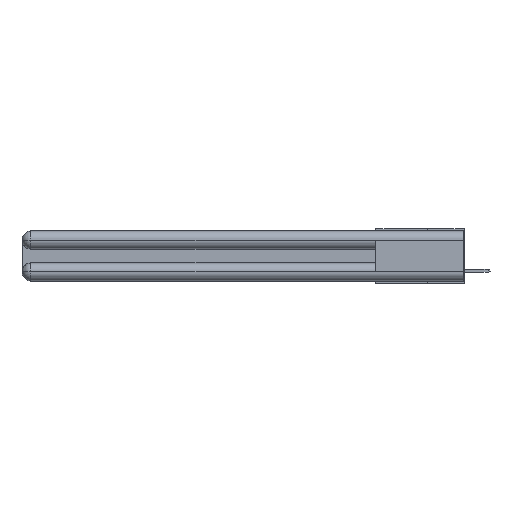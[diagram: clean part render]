
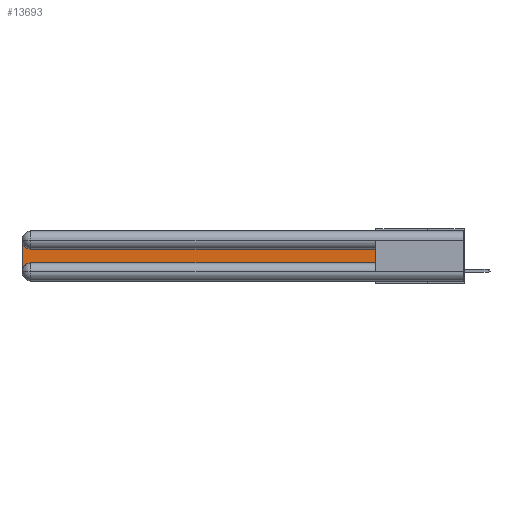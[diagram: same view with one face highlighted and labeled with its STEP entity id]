
A CAD part, left-side view. The second image highlights one B-rep face of the part: STEP entity #13693.
In plain terms, the highlighted planar face has unit normal (-1, 0, 0).
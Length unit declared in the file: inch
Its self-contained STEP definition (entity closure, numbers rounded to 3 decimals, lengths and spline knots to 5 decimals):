
#101 = CARTESIAN_POINT ( 'NONE',  ( 0.075, 2.94, -0.2175 ) ) ;
#465 = VECTOR ( 'NONE', #5358, 39.37008 ) ;
#733 = DIRECTION ( 'NONE',  ( 0., 0., -1. ) ) ;
#2989 = CARTESIAN_POINT ( 'NONE',  ( 0.075, 2.94, -0.1225 ) ) ;
#3214 = EDGE_CURVE ( 'NONE', #12078, #3903, #7138, .T. ) ;
#3518 = DIRECTION ( 'NONE',  ( 0., 0., -1. ) ) ;
#3673 = EDGE_LOOP ( 'NONE', ( #28659, #23181, #9239, #20537, #23320, #14906 ) ) ;
#3903 = VERTEX_POINT ( 'NONE', #20853 ) ;
#4995 = LINE ( 'NONE', #23506, #28482 ) ;
#5081 = DIRECTION ( 'NONE',  ( 0., 1., 0. ) ) ;
#5358 = DIRECTION ( 'NONE',  ( 0., -1., 0. ) ) ;
#6648 = EDGE_CURVE ( 'NONE', #18941, #13173, #21908, .T. ) ;
#7138 = LINE ( 'NONE', #16647, #465 ) ;
#8792 = EDGE_CURVE ( 'NONE', #3903, #18941, #16362, .T. ) ;
#9131 = CARTESIAN_POINT ( 'NONE',  ( 0.075, 3., -0.0625 ) ) ;
#9239 = ORIENTED_EDGE ( 'NONE', *, *, #23781, .T. ) ;
#9678 = DIRECTION ( 'NONE',  ( 1., 0., 0. ) ) ;
#10400 = VECTOR ( 'NONE', #26756, 39.37008 ) ;
#11608 = VERTEX_POINT ( 'NONE', #9131 ) ;
#11963 = CARTESIAN_POINT ( 'NONE',  ( 0.075, 0.6, -0.1225 ) ) ;
#12078 = VERTEX_POINT ( 'NONE', #101 ) ;
#12513 = EDGE_CURVE ( 'NONE', #13173, #11608, #28625, .T. ) ;
#12582 = DIRECTION ( 'NONE',  ( 0., 0., -1. ) ) ;
#13173 = VERTEX_POINT ( 'NONE', #2989 ) ;
#13509 = CARTESIAN_POINT ( 'NONE',  ( 0.075, 3., -0.2775 ) ) ;
#13693 = ADVANCED_FACE ( 'NONE', ( #16802 ), #25080, .F. ) ;
#14117 = CARTESIAN_POINT ( 'NONE',  ( 0.075, 3., -0.1225 ) ) ;
#14906 = ORIENTED_EDGE ( 'NONE', *, *, #8792, .T. ) ;
#16362 = LINE ( 'NONE', #20009, #10400 ) ;
#16647 = CARTESIAN_POINT ( 'NONE',  ( 0.075, 0.6, -0.2175 ) ) ;
#16802 = FACE_OUTER_BOUND ( 'NONE', #3673, .T. ) ;
#18788 = AXIS2_PLACEMENT_3D ( 'NONE', #23752, #25998, #12582 ) ;
#18941 = VERTEX_POINT ( 'NONE', #27209 ) ;
#19852 = EDGE_CURVE ( 'NONE', #23528, #12078, #25189, .T. ) ;
#20009 = CARTESIAN_POINT ( 'NONE',  ( 0.075, 0.6, -0.2175 ) ) ;
#20537 = ORIENTED_EDGE ( 'NONE', *, *, #19852, .T. ) ;
#20853 = CARTESIAN_POINT ( 'NONE',  ( 0.075, 0.6, -0.2175 ) ) ;
#21211 = VECTOR ( 'NONE', #5081, 39.37008 ) ;
#21908 = LINE ( 'NONE', #11963, #21211 ) ;
#23181 = ORIENTED_EDGE ( 'NONE', *, *, #12513, .T. ) ;
#23320 = ORIENTED_EDGE ( 'NONE', *, *, #3214, .T. ) ;
#23506 = CARTESIAN_POINT ( 'NONE',  ( 0.075, 3., -0.2175 ) ) ;
#23528 = VERTEX_POINT ( 'NONE', #13509 ) ;
#23752 = CARTESIAN_POINT ( 'NONE',  ( 0.075, 2.94, -0.2775 ) ) ;
#23781 = EDGE_CURVE ( 'NONE', #11608, #23528, #4995, .T. ) ;
#23834 = DIRECTION ( 'NONE',  ( 1., 0., 0. ) ) ;
#25080 = PLANE ( 'NONE',  #27421 ) ;
#25189 = CIRCLE ( 'NONE', #18788, 0.06 ) ;
#25719 = AXIS2_PLACEMENT_3D ( 'NONE', #25889, #23834, #3518 ) ;
#25889 = CARTESIAN_POINT ( 'NONE',  ( 0.075, 2.94, -0.0625 ) ) ;
#25998 = DIRECTION ( 'NONE',  ( 1., 0., 0. ) ) ;
#26756 = DIRECTION ( 'NONE',  ( 0., 0., 1. ) ) ;
#27209 = CARTESIAN_POINT ( 'NONE',  ( 0.075, 0.6, -0.1225 ) ) ;
#27421 = AXIS2_PLACEMENT_3D ( 'NONE', #14117, #9678, #27640 ) ;
#27640 = DIRECTION ( 'NONE',  ( 0., 0., -1. ) ) ;
#28482 = VECTOR ( 'NONE', #733, 39.37008 ) ;
#28625 = CIRCLE ( 'NONE', #25719, 0.06 ) ;
#28659 = ORIENTED_EDGE ( 'NONE', *, *, #6648, .T. ) ;
